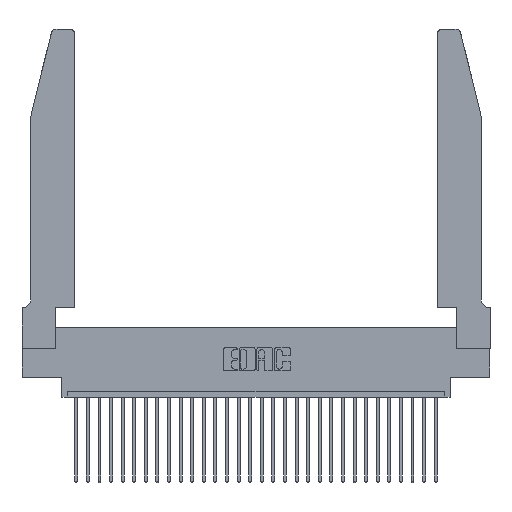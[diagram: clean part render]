
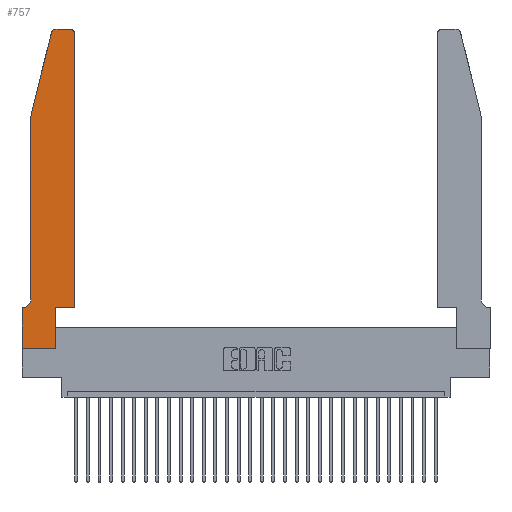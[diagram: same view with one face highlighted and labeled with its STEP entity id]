
A CAD part, top view. The second image highlights one B-rep face of the part: STEP entity #757.
In plain terms, the highlighted planar face has unit normal (0, 0, 1).
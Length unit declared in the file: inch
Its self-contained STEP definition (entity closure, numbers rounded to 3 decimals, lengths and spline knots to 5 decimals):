
#85 = CARTESIAN_POINT ( 'NONE',  ( 0.2865, 0.35, 0.37 ) ) ;
#183 = VECTOR ( 'NONE', #4853, 39.37008 ) ;
#220 = ORIENTED_EDGE ( 'NONE', *, *, #27232, .T. ) ;
#233 = CARTESIAN_POINT ( 'NONE',  ( 0.0055, 0.35, 0.37 ) ) ;
#480 = ORIENTED_EDGE ( 'NONE', *, *, #6284, .T. ) ;
#542 = EDGE_CURVE ( 'NONE', #26652, #15042, #23704, .T. ) ;
#757 = ADVANCED_FACE ( 'NONE', ( #4241 ), #25176, .T. ) ;
#1046 = VERTEX_POINT ( 'NONE', #29377 ) ;
#1115 = DIRECTION ( 'NONE',  ( 0., -1., 0. ) ) ;
#1134 = DIRECTION ( 'NONE',  ( -0.239, -0.971, 0. ) ) ;
#1341 = CARTESIAN_POINT ( 'NONE',  ( 0.4205, 2.75, 0.37 ) ) ;
#2317 = DIRECTION ( 'NONE',  ( 0., -1., 0. ) ) ;
#2738 = CARTESIAN_POINT ( 'NONE',  ( 0.25487, 2.72718, 0.37 ) ) ;
#2895 = DIRECTION ( 'NONE',  ( 0., 0., 1. ) ) ;
#3270 = AXIS2_PLACEMENT_3D ( 'NONE', #23869, #21818, #28744 ) ;
#3279 = CARTESIAN_POINT ( 'NONE',  ( 0.0755, 2., 0.37 ) ) ;
#3782 = VERTEX_POINT ( 'NONE', #2738 ) ;
#4002 = LINE ( 'NONE', #20731, #19789 ) ;
#4241 = FACE_OUTER_BOUND ( 'NONE', #4700, .T. ) ;
#4700 = EDGE_LOOP ( 'NONE', ( #27306, #14977, #19668, #27866, #220, #480, #29749, #18824, #21939, #12155, #5844, #21052 ) ) ;
#4774 = CARTESIAN_POINT ( 'NONE',  ( 0.4505, 0.35, 0.37 ) ) ;
#4853 = DIRECTION ( 'NONE',  ( 1., 0., 0. ) ) ;
#5192 = CARTESIAN_POINT ( 'NONE',  ( 0.2865, 0.35, 0.37 ) ) ;
#5327 = VERTEX_POINT ( 'NONE', #233 ) ;
#5333 = VECTOR ( 'NONE', #21199, 39.37008 ) ;
#5595 = VECTOR ( 'NONE', #8832, 39.37008 ) ;
#5820 = CARTESIAN_POINT ( 'NONE',  ( 0.284, 2.75, 0.37 ) ) ;
#5844 = ORIENTED_EDGE ( 'NONE', *, *, #10879, .T. ) ;
#6284 = EDGE_CURVE ( 'NONE', #5327, #1046, #12355, .T. ) ;
#6446 = AXIS2_PLACEMENT_3D ( 'NONE', #21377, #2895, #7308 ) ;
#7119 = EDGE_CURVE ( 'NONE', #1046, #13098, #7955, .T. ) ;
#7308 = DIRECTION ( 'NONE',  ( 1., 0., 0. ) ) ;
#7661 = CARTESIAN_POINT ( 'NONE',  ( 0.4505, 0.35, 0.37 ) ) ;
#7955 = LINE ( 'NONE', #9284, #21198 ) ;
#8455 = EDGE_CURVE ( 'NONE', #13098, #23350, #29112, .T. ) ;
#8682 = VERTEX_POINT ( 'NONE', #1341 ) ;
#8817 = AXIS2_PLACEMENT_3D ( 'NONE', #11241, #18214, #11136 ) ;
#8818 = DIRECTION ( 'NONE',  ( -1., 0., 0. ) ) ;
#8832 = DIRECTION ( 'NONE',  ( 0., 1., 0. ) ) ;
#9284 = CARTESIAN_POINT ( 'NONE',  ( 0., 0., 0.37 ) ) ;
#9455 = EDGE_CURVE ( 'NONE', #23350, #9836, #29462, .T. ) ;
#9542 = LINE ( 'NONE', #15189, #29299 ) ;
#9836 = VERTEX_POINT ( 'NONE', #85 ) ;
#9942 = CIRCLE ( 'NONE', #3270, 0.03 ) ;
#9945 = CARTESIAN_POINT ( 'NONE',  ( 0.0055, 0.42, 0.37 ) ) ;
#9979 = LINE ( 'NONE', #29608, #5595 ) ;
#10074 = AXIS2_PLACEMENT_3D ( 'NONE', #9945, #23269, #28583 ) ;
#10823 = VECTOR ( 'NONE', #1115, 39.37008 ) ;
#10879 = EDGE_CURVE ( 'NONE', #23749, #14631, #9979, .T. ) ;
#11136 = DIRECTION ( 'NONE',  ( 1., 0., 0. ) ) ;
#11241 = CARTESIAN_POINT ( 'NONE',  ( 0., 0.35, 0.37 ) ) ;
#11751 = CARTESIAN_POINT ( 'NONE',  ( 0.2865, 0., 0.37 ) ) ;
#11787 = CARTESIAN_POINT ( 'NONE',  ( 0., 0., 0.37 ) ) ;
#12155 = ORIENTED_EDGE ( 'NONE', *, *, #22840, .T. ) ;
#12355 = LINE ( 'NONE', #18576, #16397 ) ;
#12426 = CARTESIAN_POINT ( 'NONE',  ( 0.4505, 2.72, 0.37 ) ) ;
#13098 = VERTEX_POINT ( 'NONE', #11787 ) ;
#13748 = DIRECTION ( 'NONE',  ( -1., 0., 0. ) ) ;
#14631 = VERTEX_POINT ( 'NONE', #12426 ) ;
#14692 = CARTESIAN_POINT ( 'NONE',  ( 0., 0., 0.37 ) ) ;
#14977 = ORIENTED_EDGE ( 'NONE', *, *, #21716, .T. ) ;
#15042 = VERTEX_POINT ( 'NONE', #30335 ) ;
#15189 = CARTESIAN_POINT ( 'NONE',  ( 0.0755, 2., 0.37 ) ) ;
#15928 = LINE ( 'NONE', #4774, #5333 ) ;
#16397 = VECTOR ( 'NONE', #13748, 39.37008 ) ;
#16752 = CIRCLE ( 'NONE', #6446, 0.03 ) ;
#18214 = DIRECTION ( 'NONE',  ( 0., 0., 1. ) ) ;
#18576 = CARTESIAN_POINT ( 'NONE',  ( 0.0755, 0.35, 0.37 ) ) ;
#18824 = ORIENTED_EDGE ( 'NONE', *, *, #8455, .T. ) ;
#19143 = EDGE_CURVE ( 'NONE', #14631, #8682, #9942, .T. ) ;
#19668 = ORIENTED_EDGE ( 'NONE', *, *, #25152, .T. ) ;
#19789 = VECTOR ( 'NONE', #8818, 39.37008 ) ;
#20629 = CIRCLE ( 'NONE', #10074, 0.07 ) ;
#20731 = CARTESIAN_POINT ( 'NONE',  ( 0.2605, 2.75, 0.37 ) ) ;
#21052 = ORIENTED_EDGE ( 'NONE', *, *, #19143, .T. ) ;
#21198 = VECTOR ( 'NONE', #2317, 39.37008 ) ;
#21199 = DIRECTION ( 'NONE',  ( 1., 0., 0. ) ) ;
#21377 = CARTESIAN_POINT ( 'NONE',  ( 0.284, 2.72, 0.37 ) ) ;
#21716 = EDGE_CURVE ( 'NONE', #29482, #3782, #16752, .T. ) ;
#21818 = DIRECTION ( 'NONE',  ( 0., 0., 1. ) ) ;
#21939 = ORIENTED_EDGE ( 'NONE', *, *, #9455, .T. ) ;
#22840 = EDGE_CURVE ( 'NONE', #9836, #23749, #15928, .T. ) ;
#23269 = DIRECTION ( 'NONE',  ( 0., 0., -1. ) ) ;
#23350 = VERTEX_POINT ( 'NONE', #11751 ) ;
#23704 = LINE ( 'NONE', #3279, #10823 ) ;
#23749 = VERTEX_POINT ( 'NONE', #7661 ) ;
#23869 = CARTESIAN_POINT ( 'NONE',  ( 0.4205, 2.72, 0.37 ) ) ;
#23920 = CARTESIAN_POINT ( 'NONE',  ( 0.0755, 2., 0.37 ) ) ;
#25152 = EDGE_CURVE ( 'NONE', #3782, #26652, #9542, .T. ) ;
#25176 = PLANE ( 'NONE',  #8817 ) ;
#25808 = VECTOR ( 'NONE', #26366, 39.37008 ) ;
#26366 = DIRECTION ( 'NONE',  ( 0., 1., 0. ) ) ;
#26652 = VERTEX_POINT ( 'NONE', #23920 ) ;
#27232 = EDGE_CURVE ( 'NONE', #15042, #5327, #20629, .T. ) ;
#27306 = ORIENTED_EDGE ( 'NONE', *, *, #28670, .T. ) ;
#27866 = ORIENTED_EDGE ( 'NONE', *, *, #542, .T. ) ;
#28583 = DIRECTION ( 'NONE',  ( -1., 0., 0. ) ) ;
#28670 = EDGE_CURVE ( 'NONE', #8682, #29482, #4002, .T. ) ;
#28744 = DIRECTION ( 'NONE',  ( 1., 0., 0. ) ) ;
#29112 = LINE ( 'NONE', #14692, #183 ) ;
#29299 = VECTOR ( 'NONE', #1134, 39.37008 ) ;
#29377 = CARTESIAN_POINT ( 'NONE',  ( 0., 0.35, 0.37 ) ) ;
#29462 = LINE ( 'NONE', #5192, #25808 ) ;
#29482 = VERTEX_POINT ( 'NONE', #5820 ) ;
#29608 = CARTESIAN_POINT ( 'NONE',  ( 0.4505, 0.35, 0.37 ) ) ;
#29749 = ORIENTED_EDGE ( 'NONE', *, *, #7119, .T. ) ;
#30335 = CARTESIAN_POINT ( 'NONE',  ( 0.0755, 0.42, 0.37 ) ) ;
